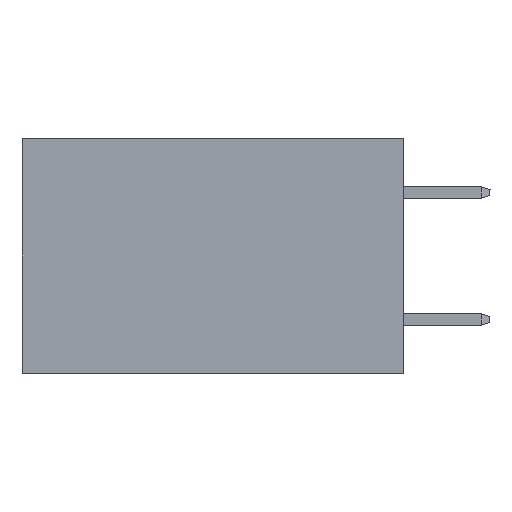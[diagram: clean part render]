
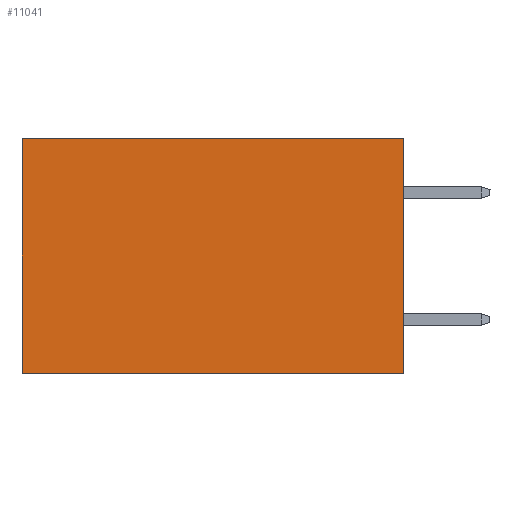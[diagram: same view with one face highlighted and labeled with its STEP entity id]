
A CAD part, left-side view. The second image highlights one B-rep face of the part: STEP entity #11041.
In plain terms, the highlighted planar face has unit normal (-1, 0, 0).
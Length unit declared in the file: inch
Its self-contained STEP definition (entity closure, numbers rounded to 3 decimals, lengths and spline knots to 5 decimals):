
#488 = CARTESIAN_POINT ( 'NONE',  ( 0.2875, 0., -0.37 ) ) ;
#1099 = DIRECTION ( 'NONE',  ( 0., 0., -1. ) ) ;
#1414 = EDGE_CURVE ( 'NONE', #13479, #13685, #9701, .T. ) ;
#1420 = ORIENTED_EDGE ( 'NONE', *, *, #1414, .F. ) ;
#1568 = CARTESIAN_POINT ( 'NONE',  ( 0.2875, 0., 0. ) ) ;
#2648 = CARTESIAN_POINT ( 'NONE',  ( 0.2875, 0., 0. ) ) ;
#3911 = LINE ( 'NONE', #2648, #10288 ) ;
#4425 = DIRECTION ( 'NONE',  ( 0., 0., -1. ) ) ;
#4499 = LINE ( 'NONE', #1568, #13620 ) ;
#6034 = EDGE_CURVE ( 'NONE', #17166, #13685, #20005, .T. ) ;
#6102 = EDGE_CURVE ( 'NONE', #13014, #17166, #3911, .T. ) ;
#6309 = ORIENTED_EDGE ( 'NONE', *, *, #17923, .F. ) ;
#6417 = AXIS2_PLACEMENT_3D ( 'NONE', #10627, #9071, #4425 ) ;
#7525 = FACE_OUTER_BOUND ( 'NONE', #8377, .T. ) ;
#7899 = DIRECTION ( 'NONE',  ( 0., 0., -1. ) ) ;
#7985 = VECTOR ( 'NONE', #1099, 39.37008 ) ;
#8158 = CARTESIAN_POINT ( 'NONE',  ( 0.2875, 0., -0.37 ) ) ;
#8377 = EDGE_LOOP ( 'NONE', ( #17977, #1420, #6309, #18534 ) ) ;
#9071 = DIRECTION ( 'NONE',  ( 1., 0., 0. ) ) ;
#9168 = PLANE ( 'NONE',  #6417 ) ;
#9701 = LINE ( 'NONE', #8158, #12756 ) ;
#10204 = DIRECTION ( 'NONE',  ( 0., 1., 0. ) ) ;
#10288 = VECTOR ( 'NONE', #10204, 39.37008 ) ;
#10627 = CARTESIAN_POINT ( 'NONE',  ( 0.2875, 0., 0. ) ) ;
#11041 = ADVANCED_FACE ( 'NONE', ( #7525 ), #9168, .F. ) ;
#12042 = CARTESIAN_POINT ( 'NONE',  ( 0.2875, 0.6, -0.37 ) ) ;
#12756 = VECTOR ( 'NONE', #12887, 39.37008 ) ;
#12887 = DIRECTION ( 'NONE',  ( 0., 1., 0. ) ) ;
#13014 = VERTEX_POINT ( 'NONE', #17204 ) ;
#13479 = VERTEX_POINT ( 'NONE', #488 ) ;
#13620 = VECTOR ( 'NONE', #7899, 39.37008 ) ;
#13685 = VERTEX_POINT ( 'NONE', #12042 ) ;
#17166 = VERTEX_POINT ( 'NONE', #19519 ) ;
#17204 = CARTESIAN_POINT ( 'NONE',  ( 0.2875, 0., 0. ) ) ;
#17923 = EDGE_CURVE ( 'NONE', #13014, #13479, #4499, .T. ) ;
#17977 = ORIENTED_EDGE ( 'NONE', *, *, #6034, .T. ) ;
#18260 = CARTESIAN_POINT ( 'NONE',  ( 0.2875, 0.6, 0. ) ) ;
#18534 = ORIENTED_EDGE ( 'NONE', *, *, #6102, .T. ) ;
#19519 = CARTESIAN_POINT ( 'NONE',  ( 0.2875, 0.6, 0. ) ) ;
#20005 = LINE ( 'NONE', #18260, #7985 ) ;
